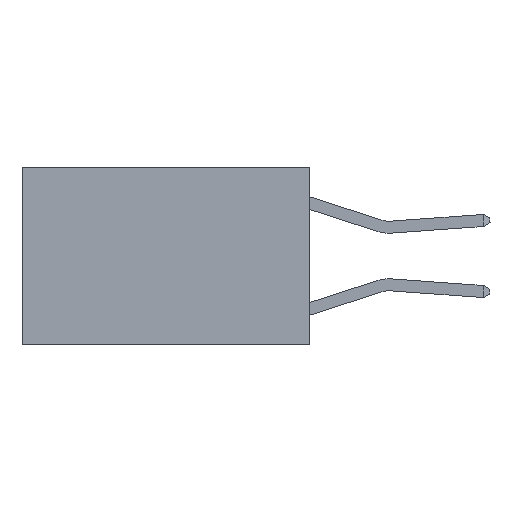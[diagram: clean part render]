
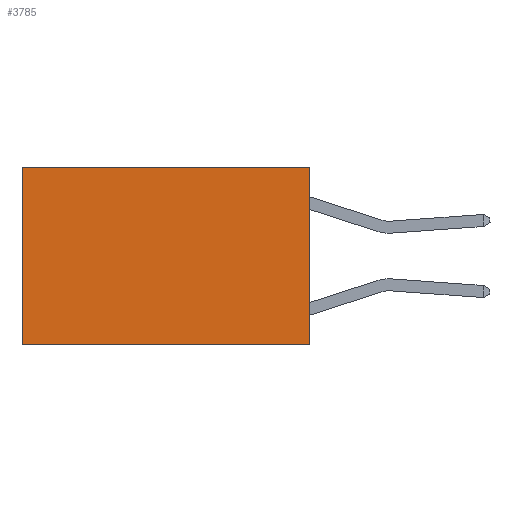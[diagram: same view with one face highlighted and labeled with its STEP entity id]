
A CAD part, left-side view. The second image highlights one B-rep face of the part: STEP entity #3785.
In plain terms, the highlighted planar face has unit normal (-1, 0, 0).
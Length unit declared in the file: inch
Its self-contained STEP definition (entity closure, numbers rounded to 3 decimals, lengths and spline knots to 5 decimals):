
#102 = VECTOR ( 'NONE', #8413, 39.37008 ) ;
#525 = VERTEX_POINT ( 'NONE', #5022 ) ;
#589 = CARTESIAN_POINT ( 'NONE',  ( 0.2625, 0., -0.37 ) ) ;
#684 = ORIENTED_EDGE ( 'NONE', *, *, #5588, .F. ) ;
#828 = AXIS2_PLACEMENT_3D ( 'NONE', #2144, #2168, #7060 ) ;
#1381 = CARTESIAN_POINT ( 'NONE',  ( 0.2625, 0., 0. ) ) ;
#1869 = CARTESIAN_POINT ( 'NONE',  ( 0.2625, 0.6, 0. ) ) ;
#2081 = VECTOR ( 'NONE', #7613, 39.37008 ) ;
#2144 = CARTESIAN_POINT ( 'NONE',  ( 0.2625, 0., 0. ) ) ;
#2168 = DIRECTION ( 'NONE',  ( 1., 0., 0. ) ) ;
#2187 = LINE ( 'NONE', #9785, #2081 ) ;
#2367 = VECTOR ( 'NONE', #5757, 39.37008 ) ;
#2449 = CARTESIAN_POINT ( 'NONE',  ( 0.2625, 0.6, -0.37 ) ) ;
#2677 = ORIENTED_EDGE ( 'NONE', *, *, #7786, .T. ) ;
#2694 = CARTESIAN_POINT ( 'NONE',  ( 0.2625, 0., 0. ) ) ;
#2804 = ORIENTED_EDGE ( 'NONE', *, *, #9957, .F. ) ;
#3785 = ADVANCED_FACE ( 'NONE', ( #7968 ), #7047, .F. ) ;
#4532 = LINE ( 'NONE', #7647, #102 ) ;
#4597 = EDGE_LOOP ( 'NONE', ( #2677, #684, #2804, #6688 ) ) ;
#4695 = LINE ( 'NONE', #1381, #9040 ) ;
#5022 = CARTESIAN_POINT ( 'NONE',  ( 0.2625, 0.6, 0. ) ) ;
#5588 = EDGE_CURVE ( 'NONE', #8523, #6243, #2187, .T. ) ;
#5757 = DIRECTION ( 'NONE',  ( 0., 0., -1. ) ) ;
#6243 = VERTEX_POINT ( 'NONE', #2449 ) ;
#6512 = LINE ( 'NONE', #1869, #2367 ) ;
#6688 = ORIENTED_EDGE ( 'NONE', *, *, #7418, .T. ) ;
#6824 = VERTEX_POINT ( 'NONE', #2694 ) ;
#6837 = DIRECTION ( 'NONE',  ( 0., 1., 0. ) ) ;
#7047 = PLANE ( 'NONE',  #828 ) ;
#7060 = DIRECTION ( 'NONE',  ( 0., 0., -1. ) ) ;
#7418 = EDGE_CURVE ( 'NONE', #6824, #525, #4695, .T. ) ;
#7613 = DIRECTION ( 'NONE',  ( 0., 1., 0. ) ) ;
#7647 = CARTESIAN_POINT ( 'NONE',  ( 0.2625, 0., 0. ) ) ;
#7786 = EDGE_CURVE ( 'NONE', #525, #6243, #6512, .T. ) ;
#7968 = FACE_OUTER_BOUND ( 'NONE', #4597, .T. ) ;
#8413 = DIRECTION ( 'NONE',  ( 0., 0., -1. ) ) ;
#8523 = VERTEX_POINT ( 'NONE', #589 ) ;
#9040 = VECTOR ( 'NONE', #6837, 39.37008 ) ;
#9785 = CARTESIAN_POINT ( 'NONE',  ( 0.2625, 0., -0.37 ) ) ;
#9957 = EDGE_CURVE ( 'NONE', #6824, #8523, #4532, .T. ) ;
